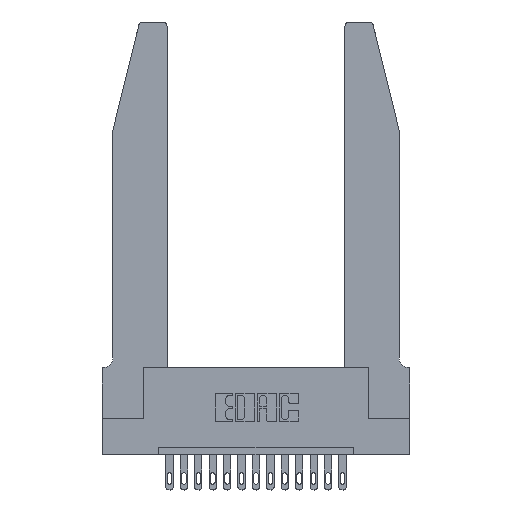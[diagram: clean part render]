
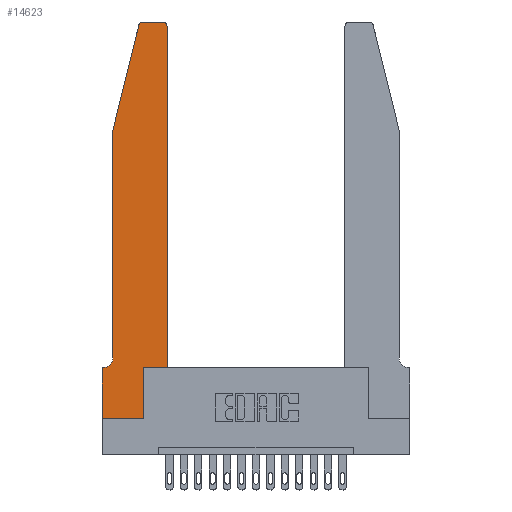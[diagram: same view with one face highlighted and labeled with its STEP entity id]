
A CAD part, top view. The second image highlights one B-rep face of the part: STEP entity #14623.
In plain terms, the highlighted planar face has unit normal (0, 0, 1).
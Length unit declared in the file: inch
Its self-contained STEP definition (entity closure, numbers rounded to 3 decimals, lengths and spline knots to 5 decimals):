
#198 = DIRECTION ( 'NONE',  ( 1., 0., 0. ) ) ;
#276 = ORIENTED_EDGE ( 'NONE', *, *, #12246, .T. ) ;
#342 = DIRECTION ( 'NONE',  ( 0., 0., -1. ) ) ;
#384 = ORIENTED_EDGE ( 'NONE', *, *, #4985, .T. ) ;
#456 = CARTESIAN_POINT ( 'NONE',  ( 0.0755, 2., 0.37 ) ) ;
#549 = EDGE_CURVE ( 'NONE', #15574, #3695, #13944, .T. ) ;
#674 = CARTESIAN_POINT ( 'NONE',  ( 0., 0., 0.37 ) ) ;
#927 = CARTESIAN_POINT ( 'NONE',  ( 0.0755, 2., 0.37 ) ) ;
#929 = EDGE_CURVE ( 'NONE', #7874, #4161, #5568, .T. ) ;
#1201 = CARTESIAN_POINT ( 'NONE',  ( 0., 0.35, 0.37 ) ) ;
#1515 = AXIS2_PLACEMENT_3D ( 'NONE', #8780, #342, #3359 ) ;
#1616 = CARTESIAN_POINT ( 'NONE',  ( 0.2865, 0.35, 0.37 ) ) ;
#1854 = CARTESIAN_POINT ( 'NONE',  ( 0.4205, 2.75, 0.37 ) ) ;
#1949 = VECTOR ( 'NONE', #10486, 39.37008 ) ;
#2090 = CARTESIAN_POINT ( 'NONE',  ( 0.4505, 0.35, 0.37 ) ) ;
#2099 = CARTESIAN_POINT ( 'NONE',  ( 0.2865, 0., 0.37 ) ) ;
#2143 = CARTESIAN_POINT ( 'NONE',  ( 0., 0., 0.37 ) ) ;
#2334 = LINE ( 'NONE', #1616, #6754 ) ;
#2523 = CARTESIAN_POINT ( 'NONE',  ( 0.284, 2.75, 0.37 ) ) ;
#2648 = DIRECTION ( 'NONE',  ( 0., 0., 1. ) ) ;
#3024 = CARTESIAN_POINT ( 'NONE',  ( 0.284, 2.72, 0.37 ) ) ;
#3300 = VECTOR ( 'NONE', #10341, 39.37008 ) ;
#3359 = DIRECTION ( 'NONE',  ( -1., 0., 0. ) ) ;
#3695 = VERTEX_POINT ( 'NONE', #456 ) ;
#3840 = VERTEX_POINT ( 'NONE', #14889 ) ;
#3846 = DIRECTION ( 'NONE',  ( 1., 0., 0. ) ) ;
#3910 = CARTESIAN_POINT ( 'NONE',  ( 0.4205, 2.72, 0.37 ) ) ;
#4161 = VERTEX_POINT ( 'NONE', #1854 ) ;
#4319 = DIRECTION ( 'NONE',  ( 0., 0., 1. ) ) ;
#4350 = VERTEX_POINT ( 'NONE', #9153 ) ;
#4369 = LINE ( 'NONE', #2143, #13199 ) ;
#4874 = AXIS2_PLACEMENT_3D ( 'NONE', #3910, #5467, #3846 ) ;
#4985 = EDGE_CURVE ( 'NONE', #14771, #16306, #8080, .T. ) ;
#5174 = DIRECTION ( 'NONE',  ( 0., 1., 0. ) ) ;
#5467 = DIRECTION ( 'NONE',  ( 0., 0., 1. ) ) ;
#5568 = CIRCLE ( 'NONE', #4874, 0.03 ) ;
#5830 = ORIENTED_EDGE ( 'NONE', *, *, #12305, .T. ) ;
#6412 = DIRECTION ( 'NONE',  ( -0.239, -0.971, 0. ) ) ;
#6754 = VECTOR ( 'NONE', #10136, 39.37008 ) ;
#7013 = VECTOR ( 'NONE', #17474, 39.37008 ) ;
#7104 = ORIENTED_EDGE ( 'NONE', *, *, #10531, .T. ) ;
#7153 = ORIENTED_EDGE ( 'NONE', *, *, #10606, .T. ) ;
#7395 = CARTESIAN_POINT ( 'NONE',  ( 0.2605, 2.75, 0.37 ) ) ;
#7637 = VECTOR ( 'NONE', #13846, 39.37008 ) ;
#7784 = ORIENTED_EDGE ( 'NONE', *, *, #11230, .T. ) ;
#7874 = VERTEX_POINT ( 'NONE', #14127 ) ;
#8080 = CIRCLE ( 'NONE', #1515, 0.07 ) ;
#8556 = EDGE_LOOP ( 'NONE', ( #15349, #276, #9466, #5830, #384, #7153, #11290, #7104, #10532, #7784, #11222, #16174 ) ) ;
#8623 = VERTEX_POINT ( 'NONE', #16939 ) ;
#8780 = CARTESIAN_POINT ( 'NONE',  ( 0.0055, 0.42, 0.37 ) ) ;
#9118 = CARTESIAN_POINT ( 'NONE',  ( 0., 0., 0.37 ) ) ;
#9153 = CARTESIAN_POINT ( 'NONE',  ( 0., 0.35, 0.37 ) ) ;
#9395 = CARTESIAN_POINT ( 'NONE',  ( 0.0055, 0.35, 0.37 ) ) ;
#9466 = ORIENTED_EDGE ( 'NONE', *, *, #549, .T. ) ;
#9691 = PLANE ( 'NONE',  #15963 ) ;
#10027 = VERTEX_POINT ( 'NONE', #2523 ) ;
#10136 = DIRECTION ( 'NONE',  ( 0., 1., 0. ) ) ;
#10218 = AXIS2_PLACEMENT_3D ( 'NONE', #3024, #4319, #198 ) ;
#10341 = DIRECTION ( 'NONE',  ( 0., -1., 0. ) ) ;
#10382 = EDGE_CURVE ( 'NONE', #4161, #10027, #16343, .T. ) ;
#10486 = DIRECTION ( 'NONE',  ( -1., 0., 0. ) ) ;
#10516 = VERTEX_POINT ( 'NONE', #674 ) ;
#10531 = EDGE_CURVE ( 'NONE', #10516, #10701, #4369, .T. ) ;
#10532 = ORIENTED_EDGE ( 'NONE', *, *, #12734, .T. ) ;
#10556 = EDGE_CURVE ( 'NONE', #8623, #7874, #16997, .T. ) ;
#10606 = EDGE_CURVE ( 'NONE', #16306, #4350, #14995, .T. ) ;
#10628 = CARTESIAN_POINT ( 'NONE',  ( 0.0755, 0.35, 0.37 ) ) ;
#10701 = VERTEX_POINT ( 'NONE', #2099 ) ;
#10914 = FACE_OUTER_BOUND ( 'NONE', #8556, .T. ) ;
#11222 = ORIENTED_EDGE ( 'NONE', *, *, #10556, .T. ) ;
#11230 = EDGE_CURVE ( 'NONE', #3840, #8623, #12950, .T. ) ;
#11290 = ORIENTED_EDGE ( 'NONE', *, *, #16691, .T. ) ;
#11729 = LINE ( 'NONE', #16601, #7637 ) ;
#12246 = EDGE_CURVE ( 'NONE', #10027, #15574, #15626, .T. ) ;
#12305 = EDGE_CURVE ( 'NONE', #3695, #14771, #11729, .T. ) ;
#12549 = VECTOR ( 'NONE', #13248, 39.37008 ) ;
#12620 = VECTOR ( 'NONE', #6412, 39.37008 ) ;
#12734 = EDGE_CURVE ( 'NONE', #10701, #3840, #2334, .T. ) ;
#12950 = LINE ( 'NONE', #2090, #7013 ) ;
#13199 = VECTOR ( 'NONE', #13236, 39.37008 ) ;
#13236 = DIRECTION ( 'NONE',  ( 1., 0., 0. ) ) ;
#13248 = DIRECTION ( 'NONE',  ( -1., 0., 0. ) ) ;
#13846 = DIRECTION ( 'NONE',  ( 0., -1., 0. ) ) ;
#13921 = DIRECTION ( 'NONE',  ( 1., 0., 0. ) ) ;
#13944 = LINE ( 'NONE', #927, #12620 ) ;
#14127 = CARTESIAN_POINT ( 'NONE',  ( 0.4505, 2.72, 0.37 ) ) ;
#14444 = CARTESIAN_POINT ( 'NONE',  ( 0.25487, 2.72718, 0.37 ) ) ;
#14623 = ADVANCED_FACE ( 'NONE', ( #10914 ), #9691, .T. ) ;
#14769 = VECTOR ( 'NONE', #5174, 39.37008 ) ;
#14771 = VERTEX_POINT ( 'NONE', #16984 ) ;
#14889 = CARTESIAN_POINT ( 'NONE',  ( 0.2865, 0.35, 0.37 ) ) ;
#14995 = LINE ( 'NONE', #10628, #1949 ) ;
#15349 = ORIENTED_EDGE ( 'NONE', *, *, #10382, .T. ) ;
#15574 = VERTEX_POINT ( 'NONE', #14444 ) ;
#15626 = CIRCLE ( 'NONE', #10218, 0.03 ) ;
#15963 = AXIS2_PLACEMENT_3D ( 'NONE', #1201, #2648, #13921 ) ;
#16174 = ORIENTED_EDGE ( 'NONE', *, *, #929, .T. ) ;
#16306 = VERTEX_POINT ( 'NONE', #9395 ) ;
#16334 = LINE ( 'NONE', #9118, #3300 ) ;
#16343 = LINE ( 'NONE', #7395, #12549 ) ;
#16601 = CARTESIAN_POINT ( 'NONE',  ( 0.0755, 2., 0.37 ) ) ;
#16691 = EDGE_CURVE ( 'NONE', #4350, #10516, #16334, .T. ) ;
#16939 = CARTESIAN_POINT ( 'NONE',  ( 0.4505, 0.35, 0.37 ) ) ;
#16984 = CARTESIAN_POINT ( 'NONE',  ( 0.0755, 0.42, 0.37 ) ) ;
#16997 = LINE ( 'NONE', #17838, #14769 ) ;
#17474 = DIRECTION ( 'NONE',  ( 1., 0., 0. ) ) ;
#17838 = CARTESIAN_POINT ( 'NONE',  ( 0.4505, 0.35, 0.37 ) ) ;
